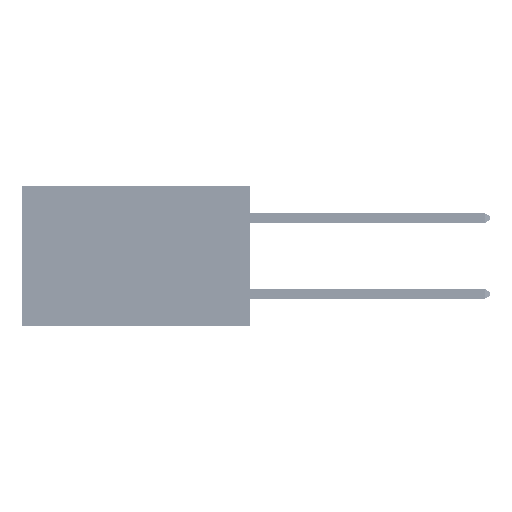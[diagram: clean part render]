
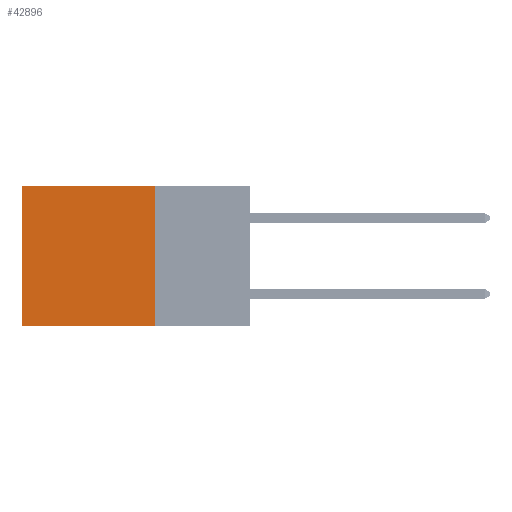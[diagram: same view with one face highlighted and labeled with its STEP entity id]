
A CAD part, left-side view. The second image highlights one B-rep face of the part: STEP entity #42896.
In plain terms, the highlighted planar face has unit normal (-1, 0, 0).
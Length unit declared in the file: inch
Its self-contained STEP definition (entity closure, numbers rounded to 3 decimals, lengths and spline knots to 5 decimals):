
#400 = EDGE_CURVE ( 'NONE', #29552, #37543, #26413, .T. ) ;
#1399 = EDGE_CURVE ( 'NONE', #37543, #29853, #28267, .T. ) ;
#2520 = ORIENTED_EDGE ( 'NONE', *, *, #4612, .F. ) ;
#4486 = ORIENTED_EDGE ( 'NONE', *, *, #37760, .F. ) ;
#4612 = EDGE_CURVE ( 'NONE', #37019, #29853, #32016, .T. ) ;
#8781 = EDGE_LOOP ( 'NONE', ( #32362, #2520, #4486, #27240 ) ) ;
#8995 = CARTESIAN_POINT ( 'NONE',  ( 0.2875, 0.6, -0.37 ) ) ;
#12652 = PLANE ( 'NONE',  #19058 ) ;
#12756 = DIRECTION ( 'NONE',  ( 0., 1., 0. ) ) ;
#13982 = DIRECTION ( 'NONE',  ( 0., 0., -1. ) ) ;
#16053 = CARTESIAN_POINT ( 'NONE',  ( 0.2875, 0.6, 0. ) ) ;
#16365 = VECTOR ( 'NONE', #40557, 39.37008 ) ;
#18438 = CARTESIAN_POINT ( 'NONE',  ( 0.2875, 0.25, 0. ) ) ;
#19058 = AXIS2_PLACEMENT_3D ( 'NONE', #27473, #24360, #28133 ) ;
#24360 = DIRECTION ( 'NONE',  ( 1., 0., 0. ) ) ;
#25171 = FACE_OUTER_BOUND ( 'NONE', #8781, .T. ) ;
#26413 = LINE ( 'NONE', #29112, #16365 ) ;
#27240 = ORIENTED_EDGE ( 'NONE', *, *, #400, .T. ) ;
#27473 = CARTESIAN_POINT ( 'NONE',  ( 0.2875, 0.25, 0. ) ) ;
#27759 = CARTESIAN_POINT ( 'NONE',  ( 0.2875, 0.25, -0.37 ) ) ;
#28133 = DIRECTION ( 'NONE',  ( 0., 0., -1. ) ) ;
#28267 = LINE ( 'NONE', #30453, #42302 ) ;
#29112 = CARTESIAN_POINT ( 'NONE',  ( 0.2875, 0.25, 0. ) ) ;
#29552 = VERTEX_POINT ( 'NONE', #18438 ) ;
#29853 = VERTEX_POINT ( 'NONE', #8995 ) ;
#30453 = CARTESIAN_POINT ( 'NONE',  ( 0.2875, 0.6, 0. ) ) ;
#30856 = VECTOR ( 'NONE', #12756, 39.37008 ) ;
#32016 = LINE ( 'NONE', #27759, #30856 ) ;
#32362 = ORIENTED_EDGE ( 'NONE', *, *, #1399, .T. ) ;
#36013 = CARTESIAN_POINT ( 'NONE',  ( 0.2875, 0.25, 0. ) ) ;
#37019 = VERTEX_POINT ( 'NONE', #39661 ) ;
#37543 = VERTEX_POINT ( 'NONE', #16053 ) ;
#37760 = EDGE_CURVE ( 'NONE', #29552, #37019, #42226, .T. ) ;
#39661 = CARTESIAN_POINT ( 'NONE',  ( 0.2875, 0.25, -0.37 ) ) ;
#40557 = DIRECTION ( 'NONE',  ( 0., 1., 0. ) ) ;
#42226 = LINE ( 'NONE', #36013, #44045 ) ;
#42302 = VECTOR ( 'NONE', #45391, 39.37008 ) ;
#42896 = ADVANCED_FACE ( 'NONE', ( #25171 ), #12652, .F. ) ;
#44045 = VECTOR ( 'NONE', #13982, 39.37008 ) ;
#45391 = DIRECTION ( 'NONE',  ( 0., 0., -1. ) ) ;
